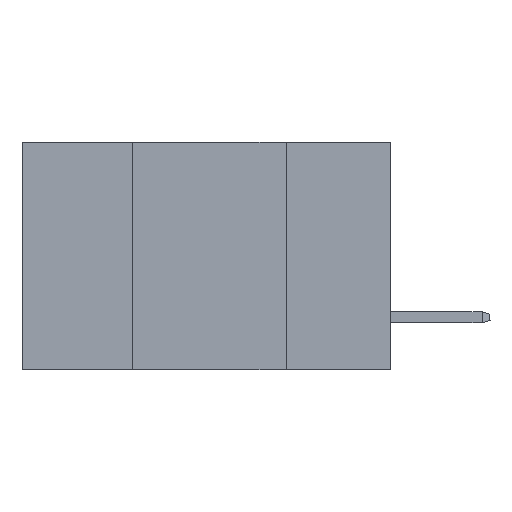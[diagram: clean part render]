
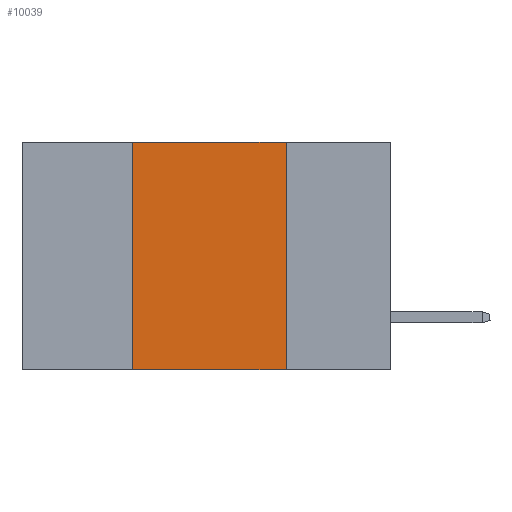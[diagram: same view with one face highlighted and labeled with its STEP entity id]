
A CAD part, left-side view. The second image highlights one B-rep face of the part: STEP entity #10039.
In plain terms, the highlighted planar face has unit normal (-1, 0, 0).
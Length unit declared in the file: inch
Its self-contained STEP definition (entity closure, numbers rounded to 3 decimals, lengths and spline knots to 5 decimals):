
#912 = LINE ( 'NONE', #12435, #7252 ) ;
#2096 = EDGE_CURVE ( 'NONE', #17236, #11159, #5270, .T. ) ;
#2124 = EDGE_CURVE ( 'NONE', #11159, #14460, #6742, .T. ) ;
#2542 = AXIS2_PLACEMENT_3D ( 'NONE', #4217, #13597, #16278 ) ;
#3052 = DIRECTION ( 'NONE',  ( 0., -1., 0. ) ) ;
#3805 = ORIENTED_EDGE ( 'NONE', *, *, #5777, .T. ) ;
#4160 = PLANE ( 'NONE',  #2542 ) ;
#4217 = CARTESIAN_POINT ( 'NONE',  ( 0., 0.6, 0. ) ) ;
#4734 = DIRECTION ( 'NONE',  ( 0., -1., 0. ) ) ;
#5270 = LINE ( 'NONE', #10290, #7801 ) ;
#5510 = CARTESIAN_POINT ( 'NONE',  ( 0., 0.42, 0. ) ) ;
#5777 = EDGE_CURVE ( 'NONE', #17210, #14460, #912, .T. ) ;
#6209 = DIRECTION ( 'NONE',  ( 0., 0., -1. ) ) ;
#6588 = ORIENTED_EDGE ( 'NONE', *, *, #8225, .F. ) ;
#6742 = LINE ( 'NONE', #14118, #13097 ) ;
#7252 = VECTOR ( 'NONE', #3052, 39.37008 ) ;
#7434 = LINE ( 'NONE', #15648, #8682 ) ;
#7656 = DIRECTION ( 'NONE',  ( 0., 0., 1. ) ) ;
#7801 = VECTOR ( 'NONE', #4734, 39.37008 ) ;
#8225 = EDGE_CURVE ( 'NONE', #17210, #17236, #7434, .T. ) ;
#8682 = VECTOR ( 'NONE', #7656, 39.37008 ) ;
#9056 = FACE_OUTER_BOUND ( 'NONE', #15038, .T. ) ;
#9077 = ORIENTED_EDGE ( 'NONE', *, *, #2096, .F. ) ;
#9356 = CARTESIAN_POINT ( 'NONE',  ( 0., 0.17, 0. ) ) ;
#10039 = ADVANCED_FACE ( 'NONE', ( #9056 ), #4160, .F. ) ;
#10290 = CARTESIAN_POINT ( 'NONE',  ( 0., 0.6, 0. ) ) ;
#11159 = VERTEX_POINT ( 'NONE', #9356 ) ;
#11933 = ORIENTED_EDGE ( 'NONE', *, *, #2124, .F. ) ;
#12435 = CARTESIAN_POINT ( 'NONE',  ( 0., 0.6, -0.37 ) ) ;
#13097 = VECTOR ( 'NONE', #6209, 39.37008 ) ;
#13597 = DIRECTION ( 'NONE',  ( 1., 0., 0. ) ) ;
#13616 = CARTESIAN_POINT ( 'NONE',  ( 0., 0.42, -0.37 ) ) ;
#14118 = CARTESIAN_POINT ( 'NONE',  ( 0., 0.17, 0. ) ) ;
#14460 = VERTEX_POINT ( 'NONE', #14872 ) ;
#14872 = CARTESIAN_POINT ( 'NONE',  ( 0., 0.17, -0.37 ) ) ;
#15038 = EDGE_LOOP ( 'NONE', ( #11933, #9077, #6588, #3805 ) ) ;
#15648 = CARTESIAN_POINT ( 'NONE',  ( 0., 0.42, 0. ) ) ;
#16278 = DIRECTION ( 'NONE',  ( 0., 0., -1. ) ) ;
#17210 = VERTEX_POINT ( 'NONE', #13616 ) ;
#17236 = VERTEX_POINT ( 'NONE', #5510 ) ;
